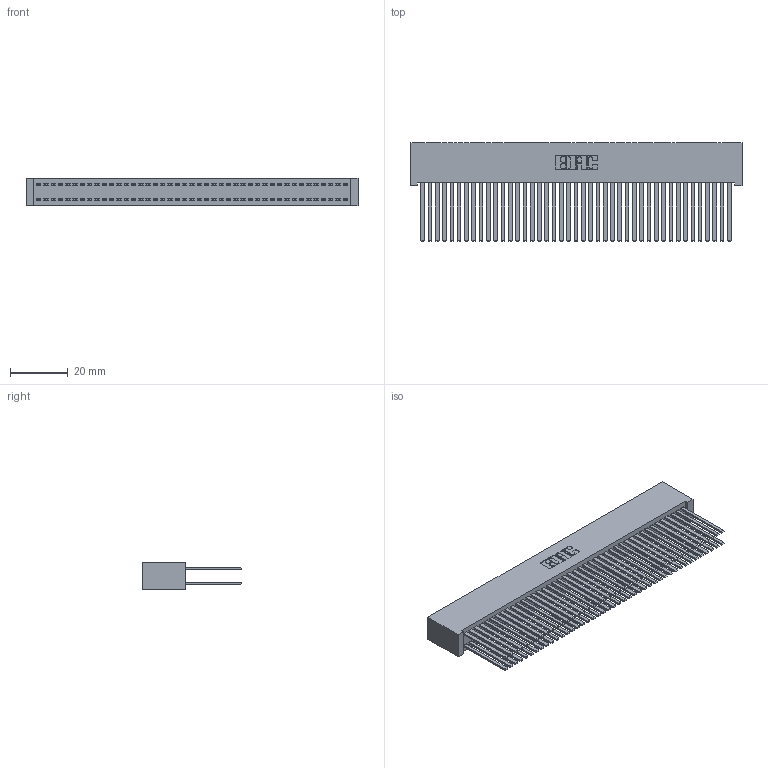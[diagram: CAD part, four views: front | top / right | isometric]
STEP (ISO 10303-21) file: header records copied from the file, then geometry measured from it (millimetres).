
FILE_DESCRIPTION (( 'STEP AP203' ), '1' );
FILE_NAME ('392-086-544-201.STEP', '2019-10-09T16:18:14', ( '' ), ( '' ), 'SwSTEP 2.0', 'SolidWorks 2016', '' );
FILE_SCHEMA (( 'CONFIG_CONTROL_DESIGN' ));
Length unit declared in the file: inch
Products named in the file (3): 342 Part_Lugless; 345-292-001_345-293-144; 392-086-544-201
Assembly tree (87 placements, depth 2):
  392-086-544-201
    342 Part_Lugless
    345-292-001_345-293-144  x86
Bounding box: 115.47 x 34.3 x 9.4 mm (x, y, z)
Volume: 12024.6 mm3; surface area: 23382.6 mm2
Topology: 87 solids, 87 shells, 4058 faces, 12057 edges, 7922 vertices
Faces by surface type: plane 2814, cylinder 1244
Entity records: 26941 total; most frequent: CARTESIAN_POINT 4458, ORIENTED_EDGE 4394, DIRECTION 3797, EDGE_CURVE 2197, VECTOR 2081, LINE 2081, VERTEX_POINT 1462, AXIS2_PLACEMENT_3D 858
